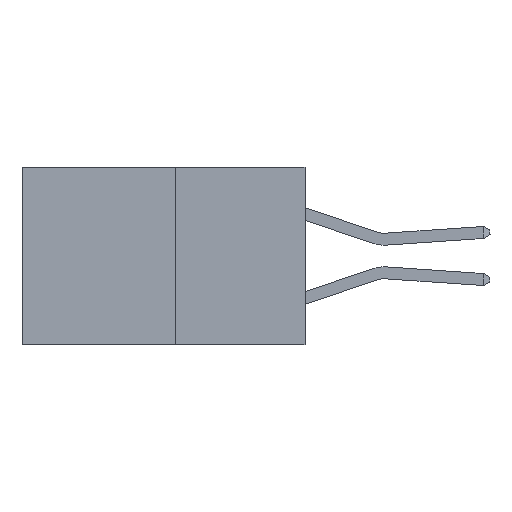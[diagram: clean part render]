
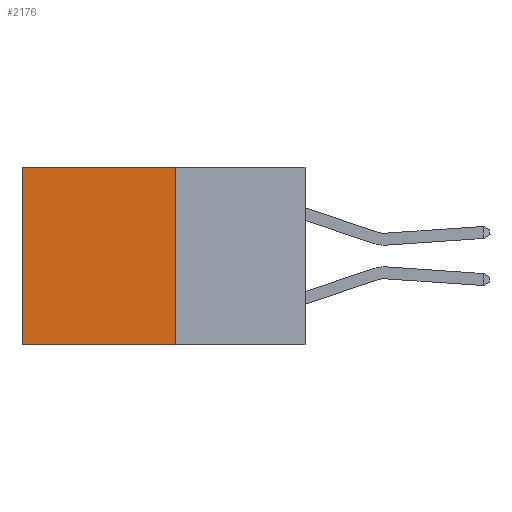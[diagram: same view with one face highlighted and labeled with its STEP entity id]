
A CAD part, left-side view. The second image highlights one B-rep face of the part: STEP entity #2176.
In plain terms, the highlighted planar face has unit normal (-1, 0, 0).
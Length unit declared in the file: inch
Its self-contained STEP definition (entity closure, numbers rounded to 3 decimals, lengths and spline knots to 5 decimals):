
#697 = EDGE_CURVE ( 'NONE', #4225, #12955, #12023, .T. ) ;
#897 = AXIS2_PLACEMENT_3D ( 'NONE', #16397, #15819, #15713 ) ;
#1394 = DIRECTION ( 'NONE',  ( 0., 0., -1. ) ) ;
#2176 = ADVANCED_FACE ( 'NONE', ( #9145 ), #8607, .F. ) ;
#2597 = EDGE_CURVE ( 'NONE', #9485, #12955, #3799, .T. ) ;
#3799 = LINE ( 'NONE', #14824, #16289 ) ;
#4180 = CARTESIAN_POINT ( 'NONE',  ( 0.277, 0.27, -0.37 ) ) ;
#4190 = CARTESIAN_POINT ( 'NONE',  ( 0.277, 0.27, -0.37 ) ) ;
#4225 = VERTEX_POINT ( 'NONE', #4180 ) ;
#4491 = DIRECTION ( 'NONE',  ( 0., 1., 0. ) ) ;
#4674 = CARTESIAN_POINT ( 'NONE',  ( 0.277, 0.27, 0. ) ) ;
#4743 = EDGE_CURVE ( 'NONE', #15193, #4225, #16641, .T. ) ;
#5737 = ORIENTED_EDGE ( 'NONE', *, *, #2597, .T. ) ;
#6413 = ORIENTED_EDGE ( 'NONE', *, *, #4743, .F. ) ;
#6910 = ORIENTED_EDGE ( 'NONE', *, *, #697, .F. ) ;
#7513 = EDGE_CURVE ( 'NONE', #15193, #9485, #16263, .T. ) ;
#8607 = PLANE ( 'NONE',  #897 ) ;
#8679 = VECTOR ( 'NONE', #12533, 39.37008 ) ;
#8688 = VECTOR ( 'NONE', #4491, 39.37008 ) ;
#9145 = FACE_OUTER_BOUND ( 'NONE', #14114, .T. ) ;
#9485 = VERTEX_POINT ( 'NONE', #11752 ) ;
#10633 = ORIENTED_EDGE ( 'NONE', *, *, #7513, .T. ) ;
#11629 = VECTOR ( 'NONE', #16278, 39.37008 ) ;
#11752 = CARTESIAN_POINT ( 'NONE',  ( 0.277, 0.59, 0. ) ) ;
#12023 = LINE ( 'NONE', #4190, #11629 ) ;
#12533 = DIRECTION ( 'NONE',  ( 0., 0., -1. ) ) ;
#12883 = CARTESIAN_POINT ( 'NONE',  ( 0.277, 0.27, -0.37 ) ) ;
#12955 = VERTEX_POINT ( 'NONE', #13577 ) ;
#13577 = CARTESIAN_POINT ( 'NONE',  ( 0.277, 0.59, -0.37 ) ) ;
#14114 = EDGE_LOOP ( 'NONE', ( #5737, #6910, #6413, #10633 ) ) ;
#14824 = CARTESIAN_POINT ( 'NONE',  ( 0.277, 0.59, -0.37 ) ) ;
#15193 = VERTEX_POINT ( 'NONE', #16663 ) ;
#15713 = DIRECTION ( 'NONE',  ( 0., 0., -1. ) ) ;
#15819 = DIRECTION ( 'NONE',  ( 1., 0., 0. ) ) ;
#16263 = LINE ( 'NONE', #4674, #8688 ) ;
#16278 = DIRECTION ( 'NONE',  ( 0., 1., 0. ) ) ;
#16289 = VECTOR ( 'NONE', #1394, 39.37008 ) ;
#16397 = CARTESIAN_POINT ( 'NONE',  ( 0.277, 0.27, -0.37 ) ) ;
#16641 = LINE ( 'NONE', #12883, #8679 ) ;
#16663 = CARTESIAN_POINT ( 'NONE',  ( 0.277, 0.27, 0. ) ) ;
